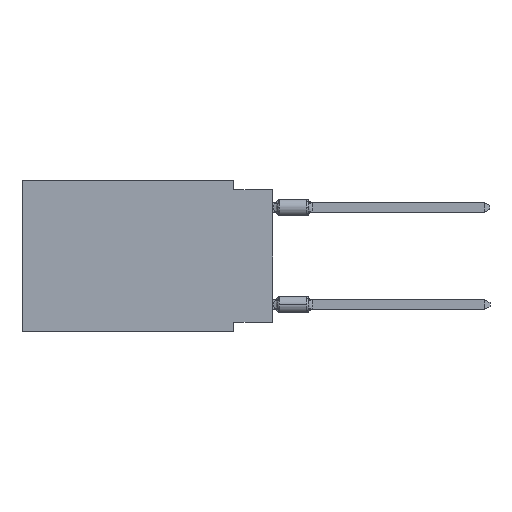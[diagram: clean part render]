
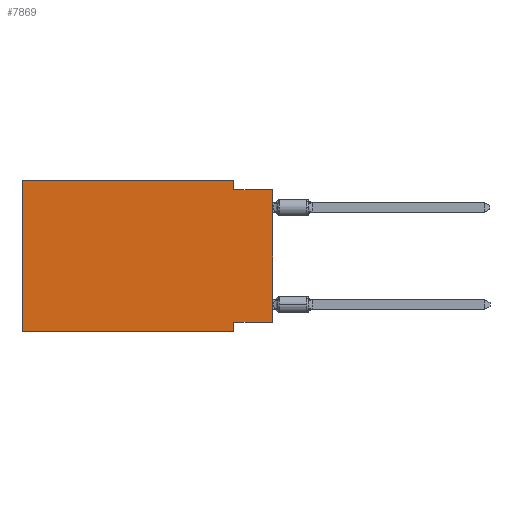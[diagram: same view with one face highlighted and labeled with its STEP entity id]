
A CAD part, left-side view. The second image highlights one B-rep face of the part: STEP entity #7869.
In plain terms, the highlighted planar face has unit normal (-1, 0, 0).
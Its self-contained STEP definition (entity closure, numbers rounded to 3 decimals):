
#373 = EDGE_CURVE ( 'NONE', #7674, #384, #15054, .T. ) ;
#384 = VERTEX_POINT ( 'NONE', #1701 ) ;
#429 = CARTESIAN_POINT ( 'NONE',  ( 0., 2.54, -9.906 ) ) ;
#1070 = CARTESIAN_POINT ( 'NONE',  ( 0., 0., -9.271 ) ) ;
#1701 = CARTESIAN_POINT ( 'NONE',  ( 0., 0., -0.635 ) ) ;
#2843 = CARTESIAN_POINT ( 'NONE',  ( 0., 16.383, 0. ) ) ;
#2859 = DIRECTION ( 'NONE',  ( 0., -1., 0. ) ) ;
#2878 = CARTESIAN_POINT ( 'NONE',  ( 0., 0., -9.271 ) ) ;
#3210 = ORIENTED_EDGE ( 'NONE', *, *, #24587, .F. ) ;
#3514 = EDGE_CURVE ( 'NONE', #5446, #23424, #13621, .T. ) ;
#4442 = CARTESIAN_POINT ( 'NONE',  ( 0., 16.383, -9.906 ) ) ;
#4645 = FACE_OUTER_BOUND ( 'NONE', #21566, .T. ) ;
#5446 = VERTEX_POINT ( 'NONE', #16567 ) ;
#6084 = CARTESIAN_POINT ( 'NONE',  ( 0., 2.54, -0.635 ) ) ;
#6277 = CARTESIAN_POINT ( 'NONE',  ( 0., 2.54, 0. ) ) ;
#6658 = ORIENTED_EDGE ( 'NONE', *, *, #13830, .T. ) ;
#6904 = VECTOR ( 'NONE', #13751, 1000. ) ;
#7248 = CARTESIAN_POINT ( 'NONE',  ( 0., 16.383, -9.906 ) ) ;
#7630 = AXIS2_PLACEMENT_3D ( 'NONE', #2843, #12551, #10608 ) ;
#7645 = CARTESIAN_POINT ( 'NONE',  ( 0., 0., -0.635 ) ) ;
#7674 = VERTEX_POINT ( 'NONE', #6084 ) ;
#7869 = ADVANCED_FACE ( 'NONE', ( #4645 ), #10729, .F. ) ;
#9207 = VERTEX_POINT ( 'NONE', #19386 ) ;
#9859 = EDGE_CURVE ( 'NONE', #10601, #9207, #23134, .T. ) ;
#10601 = VERTEX_POINT ( 'NONE', #4442 ) ;
#10608 = DIRECTION ( 'NONE',  ( 0., 0., -1. ) ) ;
#10729 = PLANE ( 'NONE',  #7630 ) ;
#10845 = VECTOR ( 'NONE', #14680, 1000. ) ;
#11650 = ORIENTED_EDGE ( 'NONE', *, *, #373, .F. ) ;
#12468 = LINE ( 'NONE', #1070, #10845 ) ;
#12551 = DIRECTION ( 'NONE',  ( 1., 0., 0. ) ) ;
#12873 = CARTESIAN_POINT ( 'NONE',  ( 0., 16.383, 0. ) ) ;
#13394 = LINE ( 'NONE', #12873, #23388 ) ;
#13588 = ORIENTED_EDGE ( 'NONE', *, *, #23545, .F. ) ;
#13621 = LINE ( 'NONE', #19591, #6904 ) ;
#13751 = DIRECTION ( 'NONE',  ( 0., 0., -1. ) ) ;
#13830 = EDGE_CURVE ( 'NONE', #17488, #384, #18795, .T. ) ;
#14082 = ORIENTED_EDGE ( 'NONE', *, *, #9859, .F. ) ;
#14680 = DIRECTION ( 'NONE',  ( 0., 1., 0. ) ) ;
#15036 = EDGE_CURVE ( 'NONE', #10601, #23424, #20849, .T. ) ;
#15054 = LINE ( 'NONE', #7645, #15688 ) ;
#15086 = DIRECTION ( 'NONE',  ( 0., -1., 0. ) ) ;
#15688 = VECTOR ( 'NONE', #23312, 1000. ) ;
#16465 = DIRECTION ( 'NONE',  ( 0., 0., 1. ) ) ;
#16567 = CARTESIAN_POINT ( 'NONE',  ( 0., 2.54, -9.271 ) ) ;
#16589 = DIRECTION ( 'NONE',  ( 0., 0., 1. ) ) ;
#16689 = VECTOR ( 'NONE', #2859, 1000. ) ;
#17488 = VERTEX_POINT ( 'NONE', #2878 ) ;
#17830 = VECTOR ( 'NONE', #24274, 1000. ) ;
#18422 = ORIENTED_EDGE ( 'NONE', *, *, #3514, .F. ) ;
#18457 = VERTEX_POINT ( 'NONE', #25429 ) ;
#18795 = LINE ( 'NONE', #20475, #23352 ) ;
#19386 = CARTESIAN_POINT ( 'NONE',  ( 0., 16.383, 0. ) ) ;
#19591 = CARTESIAN_POINT ( 'NONE',  ( 0., 2.54, -9.906 ) ) ;
#20475 = CARTESIAN_POINT ( 'NONE',  ( 0., 0., 0. ) ) ;
#20811 = EDGE_CURVE ( 'NONE', #9207, #18457, #13394, .T. ) ;
#20849 = LINE ( 'NONE', #7248, #16689 ) ;
#21379 = VECTOR ( 'NONE', #16465, 1000. ) ;
#21566 = EDGE_LOOP ( 'NONE', ( #6658, #11650, #3210, #23961, #14082, #24136, #18422, #13588 ) ) ;
#22072 = LINE ( 'NONE', #6277, #17830 ) ;
#22525 = CARTESIAN_POINT ( 'NONE',  ( 0., 16.383, 0. ) ) ;
#23134 = LINE ( 'NONE', #22525, #21379 ) ;
#23312 = DIRECTION ( 'NONE',  ( 0., -1., 0. ) ) ;
#23352 = VECTOR ( 'NONE', #16589, 1000. ) ;
#23388 = VECTOR ( 'NONE', #15086, 1000. ) ;
#23424 = VERTEX_POINT ( 'NONE', #429 ) ;
#23545 = EDGE_CURVE ( 'NONE', #17488, #5446, #12468, .T. ) ;
#23961 = ORIENTED_EDGE ( 'NONE', *, *, #20811, .F. ) ;
#24136 = ORIENTED_EDGE ( 'NONE', *, *, #15036, .T. ) ;
#24274 = DIRECTION ( 'NONE',  ( 0., 0., -1. ) ) ;
#24587 = EDGE_CURVE ( 'NONE', #18457, #7674, #22072, .T. ) ;
#25429 = CARTESIAN_POINT ( 'NONE',  ( 0., 2.54, 0. ) ) ;
